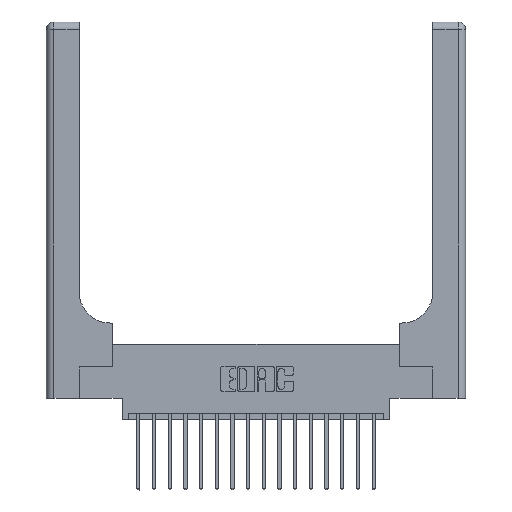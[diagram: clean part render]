
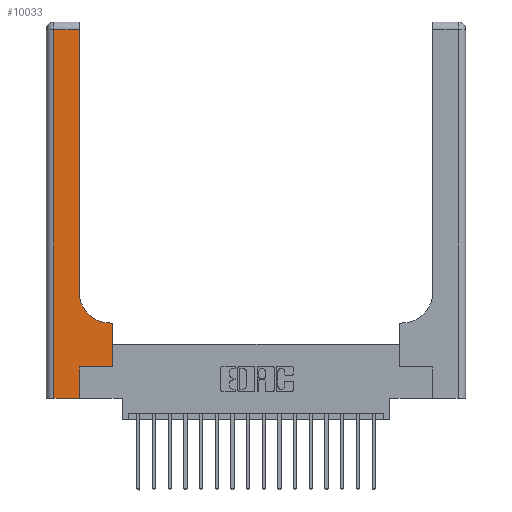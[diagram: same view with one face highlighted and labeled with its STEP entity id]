
A CAD part, top view. The second image highlights one B-rep face of the part: STEP entity #10033.
In plain terms, the highlighted planar face has unit normal (0, 0, 1).
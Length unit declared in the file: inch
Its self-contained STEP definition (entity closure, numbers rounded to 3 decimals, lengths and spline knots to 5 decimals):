
#74 = VERTEX_POINT ( 'NONE', #5563 ) ;
#293 = CARTESIAN_POINT ( 'NONE',  ( 0.26, 0.6, 0.37 ) ) ;
#470 = LINE ( 'NONE', #16695, #15421 ) ;
#517 = CARTESIAN_POINT ( 'NONE',  ( 0.26, 3., 0.37 ) ) ;
#769 = ORIENTED_EDGE ( 'NONE', *, *, #15818, .T. ) ;
#1143 = CIRCLE ( 'NONE', #3168, 0.25 ) ;
#1234 = DIRECTION ( 'NONE',  ( 0., 0., -1. ) ) ;
#1408 = CARTESIAN_POINT ( 'NONE',  ( 0.528, 0.25, 0.37 ) ) ;
#1576 = VERTEX_POINT ( 'NONE', #10532 ) ;
#2132 = CARTESIAN_POINT ( 'NONE',  ( 0.51, 0.6, 0.37 ) ) ;
#2915 = EDGE_LOOP ( 'NONE', ( #7938, #15537, #18762, #8921, #6110, #17476, #769, #10060, #5958 ) ) ;
#3046 = CARTESIAN_POINT ( 'NONE',  ( 0.06, 3., 0.37 ) ) ;
#3157 = PLANE ( 'NONE',  #12808 ) ;
#3168 = AXIS2_PLACEMENT_3D ( 'NONE', #10207, #1234, #11709 ) ;
#3387 = EDGE_CURVE ( 'NONE', #10655, #3990, #13244, .T. ) ;
#3990 = VERTEX_POINT ( 'NONE', #5210 ) ;
#4065 = DIRECTION ( 'NONE',  ( 1., 0., 0. ) ) ;
#4152 = DIRECTION ( 'NONE',  ( 1., 0., 0. ) ) ;
#4576 = DIRECTION ( 'NONE',  ( 0., -1., 0. ) ) ;
#5210 = CARTESIAN_POINT ( 'NONE',  ( 0.528, 0.25, 0.37 ) ) ;
#5359 = VECTOR ( 'NONE', #4065, 39.37008 ) ;
#5538 = DIRECTION ( 'NONE',  ( 0., 1., 0. ) ) ;
#5563 = CARTESIAN_POINT ( 'NONE',  ( 0.26, 0.85, 0.37 ) ) ;
#5749 = CARTESIAN_POINT ( 'NONE',  ( 0.528, 0.6, 0.37 ) ) ;
#5958 = ORIENTED_EDGE ( 'NONE', *, *, #18163, .T. ) ;
#6110 = ORIENTED_EDGE ( 'NONE', *, *, #10473, .T. ) ;
#6218 = CARTESIAN_POINT ( 'NONE',  ( 0., 3., 0.37 ) ) ;
#6284 = EDGE_CURVE ( 'NONE', #18162, #8023, #8502, .T. ) ;
#6333 = DIRECTION ( 'NONE',  ( -1., 0., 0. ) ) ;
#6861 = FACE_OUTER_BOUND ( 'NONE', #2915, .T. ) ;
#7267 = EDGE_CURVE ( 'NONE', #1576, #15898, #470, .T. ) ;
#7379 = EDGE_CURVE ( 'NONE', #74, #1576, #18397, .T. ) ;
#7418 = CARTESIAN_POINT ( 'NONE',  ( 0.265, 0.25, 0.37 ) ) ;
#7682 = DIRECTION ( 'NONE',  ( 0., 0., -1. ) ) ;
#7938 = ORIENTED_EDGE ( 'NONE', *, *, #7379, .T. ) ;
#8023 = VERTEX_POINT ( 'NONE', #2132 ) ;
#8368 = CARTESIAN_POINT ( 'NONE',  ( 0.06, 0., 0.37 ) ) ;
#8502 = LINE ( 'NONE', #293, #12453 ) ;
#8510 = CARTESIAN_POINT ( 'NONE',  ( 0.265, 0., 0.37 ) ) ;
#8878 = DIRECTION ( 'NONE',  ( 0., 1., 0. ) ) ;
#8921 = ORIENTED_EDGE ( 'NONE', *, *, #12454, .T. ) ;
#9126 = CARTESIAN_POINT ( 'NONE',  ( 0.06, 2.94, 0.37 ) ) ;
#9303 = DIRECTION ( 'NONE',  ( -1., 0., 0. ) ) ;
#9937 = VECTOR ( 'NONE', #4576, 39.37008 ) ;
#10033 = ADVANCED_FACE ( 'NONE', ( #6861 ), #3157, .F. ) ;
#10060 = ORIENTED_EDGE ( 'NONE', *, *, #6284, .T. ) ;
#10207 = CARTESIAN_POINT ( 'NONE',  ( 0.51, 0.85, 0.37 ) ) ;
#10397 = VERTEX_POINT ( 'NONE', #14286 ) ;
#10473 = EDGE_CURVE ( 'NONE', #10397, #10655, #16098, .T. ) ;
#10532 = CARTESIAN_POINT ( 'NONE',  ( 0.26, 2.94, 0.37 ) ) ;
#10655 = VERTEX_POINT ( 'NONE', #7418 ) ;
#11007 = DIRECTION ( 'NONE',  ( 0., 1., 0. ) ) ;
#11602 = CARTESIAN_POINT ( 'NONE',  ( 0., 0., 0.37 ) ) ;
#11709 = DIRECTION ( 'NONE',  ( 1., 0., 0. ) ) ;
#12156 = VECTOR ( 'NONE', #5538, 39.37008 ) ;
#12240 = VERTEX_POINT ( 'NONE', #8368 ) ;
#12453 = VECTOR ( 'NONE', #6333, 39.37008 ) ;
#12454 = EDGE_CURVE ( 'NONE', #12240, #10397, #15551, .T. ) ;
#12808 = AXIS2_PLACEMENT_3D ( 'NONE', #6218, #7682, #18013 ) ;
#13244 = LINE ( 'NONE', #15918, #5359 ) ;
#13718 = EDGE_CURVE ( 'NONE', #15898, #12240, #17334, .T. ) ;
#14286 = CARTESIAN_POINT ( 'NONE',  ( 0.265, 0., 0.37 ) ) ;
#14793 = VECTOR ( 'NONE', #8878, 39.37008 ) ;
#15245 = LINE ( 'NONE', #1408, #14793 ) ;
#15421 = VECTOR ( 'NONE', #9303, 39.37008 ) ;
#15537 = ORIENTED_EDGE ( 'NONE', *, *, #7267, .T. ) ;
#15551 = LINE ( 'NONE', #11602, #18997 ) ;
#15818 = EDGE_CURVE ( 'NONE', #3990, #18162, #15245, .T. ) ;
#15898 = VERTEX_POINT ( 'NONE', #9126 ) ;
#15918 = CARTESIAN_POINT ( 'NONE',  ( 0.265, 0.25, 0.37 ) ) ;
#16098 = LINE ( 'NONE', #8510, #12156 ) ;
#16695 = CARTESIAN_POINT ( 'NONE',  ( 0., 2.94, 0.37 ) ) ;
#17334 = LINE ( 'NONE', #3046, #9937 ) ;
#17472 = VECTOR ( 'NONE', #11007, 39.37008 ) ;
#17476 = ORIENTED_EDGE ( 'NONE', *, *, #3387, .T. ) ;
#18013 = DIRECTION ( 'NONE',  ( -1., 0., 0. ) ) ;
#18162 = VERTEX_POINT ( 'NONE', #5749 ) ;
#18163 = EDGE_CURVE ( 'NONE', #8023, #74, #1143, .T. ) ;
#18397 = LINE ( 'NONE', #517, #17472 ) ;
#18762 = ORIENTED_EDGE ( 'NONE', *, *, #13718, .T. ) ;
#18997 = VECTOR ( 'NONE', #4152, 39.37008 ) ;
